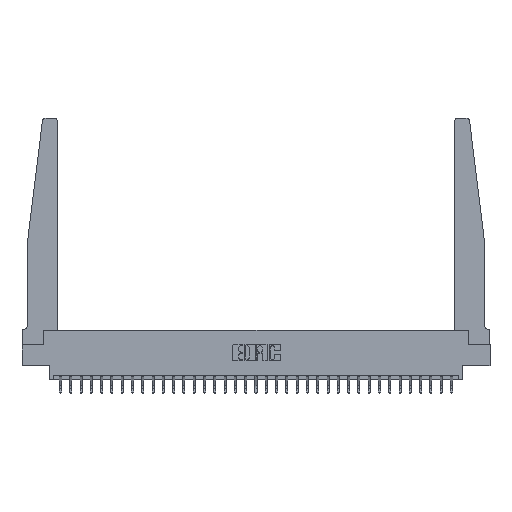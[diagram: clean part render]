
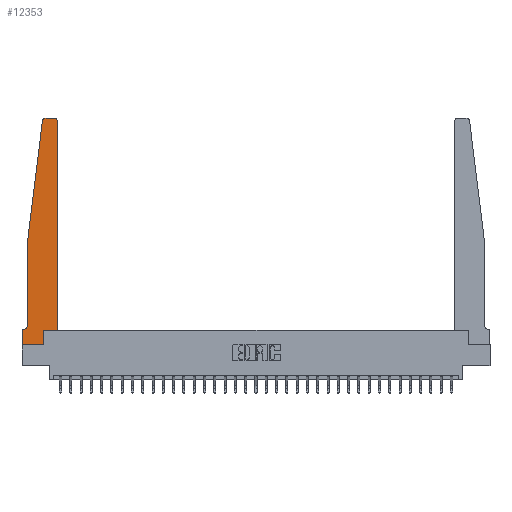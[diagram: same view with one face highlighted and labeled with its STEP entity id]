
A CAD part, top view. The second image highlights one B-rep face of the part: STEP entity #12353.
In plain terms, the highlighted planar face has unit normal (0, 0, 1).
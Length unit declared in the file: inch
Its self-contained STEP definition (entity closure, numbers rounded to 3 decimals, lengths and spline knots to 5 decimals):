
#47 = ORIENTED_EDGE ( 'NONE', *, *, #7000, .T. ) ;
#243 = ORIENTED_EDGE ( 'NONE', *, *, #26244, .T. ) ;
#430 = VECTOR ( 'NONE', #24213, 39.37008 ) ;
#449 = DIRECTION ( 'NONE',  ( 0., -1., 0. ) ) ;
#778 = EDGE_LOOP ( 'NONE', ( #21129, #3156, #21333, #22045, #10022, #23359, #243, #11355, #15871, #47, #26475, #19771 ) ) ;
#1984 = LINE ( 'NONE', #21042, #26753 ) ;
#2127 = LINE ( 'NONE', #22741, #14186 ) ;
#2691 = CARTESIAN_POINT ( 'NONE',  ( 0.25, 2.75, 0.37 ) ) ;
#3156 = ORIENTED_EDGE ( 'NONE', *, *, #30887, .T. ) ;
#3251 = CIRCLE ( 'NONE', #4327, 0.03 ) ;
#3439 = DIRECTION ( 'NONE',  ( 1., 0., 0. ) ) ;
#3648 = VECTOR ( 'NONE', #13017, 39.37008 ) ;
#3734 = EDGE_CURVE ( 'NONE', #11732, #20242, #5714, .T. ) ;
#3925 = EDGE_CURVE ( 'NONE', #22985, #16620, #13240, .T. ) ;
#4081 = EDGE_CURVE ( 'NONE', #24904, #5507, #28531, .T. ) ;
#4327 = AXIS2_PLACEMENT_3D ( 'NONE', #21396, #6992, #23773 ) ;
#5158 = LINE ( 'NONE', #10499, #3648 ) ;
#5507 = VERTEX_POINT ( 'NONE', #8179 ) ;
#5714 = LINE ( 'NONE', #30747, #11353 ) ;
#5748 = DIRECTION ( 'NONE',  ( 0., 0., -1. ) ) ;
#5939 = DIRECTION ( 'NONE',  ( 0., -1., 0. ) ) ;
#6181 = CARTESIAN_POINT ( 'NONE',  ( 0.065, 0.1875, 0.37 ) ) ;
#6825 = CARTESIAN_POINT ( 'NONE',  ( 0.425, 0.18, 0.37 ) ) ;
#6992 = DIRECTION ( 'NONE',  ( 0., 0., 1. ) ) ;
#7000 = EDGE_CURVE ( 'NONE', #16755, #11732, #12022, .T. ) ;
#7889 = CARTESIAN_POINT ( 'NONE',  ( 0.065, 0.2375, 0.37 ) ) ;
#8179 = CARTESIAN_POINT ( 'NONE',  ( 0.015, 0.1875, 0.37 ) ) ;
#8706 = CARTESIAN_POINT ( 'NONE',  ( 0., 0., 0.37 ) ) ;
#8783 = CARTESIAN_POINT ( 'NONE',  ( 0.425, 2.72, 0.37 ) ) ;
#9354 = DIRECTION ( 'NONE',  ( 0., 1., 0. ) ) ;
#9957 = LINE ( 'NONE', #28698, #21990 ) ;
#10022 = ORIENTED_EDGE ( 'NONE', *, *, #4081, .T. ) ;
#10145 = EDGE_CURVE ( 'NONE', #14494, #27181, #9957, .T. ) ;
#10499 = CARTESIAN_POINT ( 'NONE',  ( 0.2605, 0.18, 0.37 ) ) ;
#10527 = VECTOR ( 'NONE', #28378, 39.37008 ) ;
#10537 = EDGE_CURVE ( 'NONE', #5507, #12100, #24162, .T. ) ;
#10771 = DIRECTION ( 'NONE',  ( 0., 0., 1. ) ) ;
#11057 = VECTOR ( 'NONE', #449, 39.37008 ) ;
#11120 = CARTESIAN_POINT ( 'NONE',  ( 0.065, 1.25, 0.37 ) ) ;
#11353 = VECTOR ( 'NONE', #9354, 39.37008 ) ;
#11355 = ORIENTED_EDGE ( 'NONE', *, *, #26587, .T. ) ;
#11521 = CARTESIAN_POINT ( 'NONE',  ( 0.395, 2.75, 0.37 ) ) ;
#11732 = VERTEX_POINT ( 'NONE', #20316 ) ;
#12022 = LINE ( 'NONE', #6825, #10527 ) ;
#12100 = VERTEX_POINT ( 'NONE', #26307 ) ;
#12229 = CARTESIAN_POINT ( 'NONE',  ( 0.27653, 2.75, 0.37 ) ) ;
#12353 = ADVANCED_FACE ( 'NONE', ( #14746 ), #29614, .T. ) ;
#13017 = DIRECTION ( 'NONE',  ( 0., 1., 0. ) ) ;
#13240 = LINE ( 'NONE', #2691, #430 ) ;
#13329 = LINE ( 'NONE', #29149, #11057 ) ;
#13464 = CIRCLE ( 'NONE', #20272, 0.03 ) ;
#13973 = VERTEX_POINT ( 'NONE', #23510 ) ;
#14186 = VECTOR ( 'NONE', #5939, 39.37008 ) ;
#14248 = CARTESIAN_POINT ( 'NONE',  ( 0.24675, 2.72367, 0.37 ) ) ;
#14494 = VERTEX_POINT ( 'NONE', #14248 ) ;
#14746 = FACE_OUTER_BOUND ( 'NONE', #778, .T. ) ;
#15154 = CARTESIAN_POINT ( 'NONE',  ( 0.2605, 0.18, 0.37 ) ) ;
#15855 = DIRECTION ( 'NONE',  ( -1., 0., 0. ) ) ;
#15871 = ORIENTED_EDGE ( 'NONE', *, *, #22766, .T. ) ;
#16238 = EDGE_CURVE ( 'NONE', #27181, #24904, #2127, .T. ) ;
#16620 = VERTEX_POINT ( 'NONE', #12229 ) ;
#16755 = VERTEX_POINT ( 'NONE', #15154 ) ;
#17864 = DIRECTION ( 'NONE',  ( 0., 0., 1. ) ) ;
#18722 = DIRECTION ( 'NONE',  ( 1., 0., 0. ) ) ;
#19231 = DIRECTION ( 'NONE',  ( -0.122, -0.992, 0. ) ) ;
#19771 = ORIENTED_EDGE ( 'NONE', *, *, #23049, .T. ) ;
#20149 = CARTESIAN_POINT ( 'NONE',  ( 0.015, 0.2375, 0.37 ) ) ;
#20242 = VERTEX_POINT ( 'NONE', #8783 ) ;
#20272 = AXIS2_PLACEMENT_3D ( 'NONE', #25102, #10771, #27494 ) ;
#20316 = CARTESIAN_POINT ( 'NONE',  ( 0.425, 0.18, 0.37 ) ) ;
#21042 = CARTESIAN_POINT ( 'NONE',  ( 0., 0., 0.37 ) ) ;
#21129 = ORIENTED_EDGE ( 'NONE', *, *, #3925, .T. ) ;
#21333 = ORIENTED_EDGE ( 'NONE', *, *, #10145, .T. ) ;
#21396 = CARTESIAN_POINT ( 'NONE',  ( 0.395, 2.72, 0.37 ) ) ;
#21580 = VERTEX_POINT ( 'NONE', #8706 ) ;
#21990 = VECTOR ( 'NONE', #19231, 39.37008 ) ;
#22045 = ORIENTED_EDGE ( 'NONE', *, *, #16238, .T. ) ;
#22561 = DIRECTION ( 'NONE',  ( -1., 0., 0. ) ) ;
#22741 = CARTESIAN_POINT ( 'NONE',  ( 0.065, 1.25, 0.37 ) ) ;
#22766 = EDGE_CURVE ( 'NONE', #13973, #16755, #5158, .T. ) ;
#22985 = VERTEX_POINT ( 'NONE', #11521 ) ;
#23049 = EDGE_CURVE ( 'NONE', #20242, #22985, #3251, .T. ) ;
#23359 = ORIENTED_EDGE ( 'NONE', *, *, #10537, .T. ) ;
#23510 = CARTESIAN_POINT ( 'NONE',  ( 0.2605, 0., 0.37 ) ) ;
#23773 = DIRECTION ( 'NONE',  ( 1., 0., 0. ) ) ;
#24053 = AXIS2_PLACEMENT_3D ( 'NONE', #20149, #5748, #22561 ) ;
#24162 = LINE ( 'NONE', #6181, #29727 ) ;
#24213 = DIRECTION ( 'NONE',  ( -1., 0., 0. ) ) ;
#24904 = VERTEX_POINT ( 'NONE', #7889 ) ;
#24949 = CARTESIAN_POINT ( 'NONE',  ( 0., 0.1875, 0.37 ) ) ;
#25102 = CARTESIAN_POINT ( 'NONE',  ( 0.27653, 2.72, 0.37 ) ) ;
#26244 = EDGE_CURVE ( 'NONE', #12100, #21580, #13329, .T. ) ;
#26307 = CARTESIAN_POINT ( 'NONE',  ( 0., 0.1875, 0.37 ) ) ;
#26475 = ORIENTED_EDGE ( 'NONE', *, *, #3734, .T. ) ;
#26587 = EDGE_CURVE ( 'NONE', #21580, #13973, #1984, .T. ) ;
#26753 = VECTOR ( 'NONE', #18722, 39.37008 ) ;
#27181 = VERTEX_POINT ( 'NONE', #11120 ) ;
#27494 = DIRECTION ( 'NONE',  ( 1., 0., 0. ) ) ;
#28378 = DIRECTION ( 'NONE',  ( 1., 0., 0. ) ) ;
#28531 = CIRCLE ( 'NONE', #24053, 0.05 ) ;
#28698 = CARTESIAN_POINT ( 'NONE',  ( 0.065, 1.25, 0.37 ) ) ;
#28833 = AXIS2_PLACEMENT_3D ( 'NONE', #24949, #17864, #3439 ) ;
#29149 = CARTESIAN_POINT ( 'NONE',  ( 0., 0., 0.37 ) ) ;
#29614 = PLANE ( 'NONE',  #28833 ) ;
#29727 = VECTOR ( 'NONE', #15855, 39.37008 ) ;
#30747 = CARTESIAN_POINT ( 'NONE',  ( 0.425, 0.18, 0.37 ) ) ;
#30887 = EDGE_CURVE ( 'NONE', #16620, #14494, #13464, .T. ) ;
